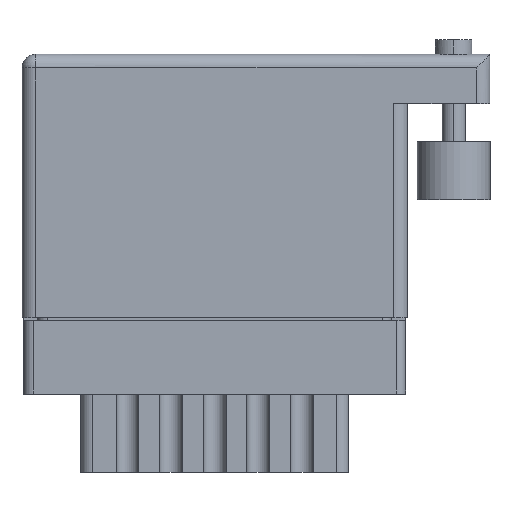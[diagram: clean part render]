
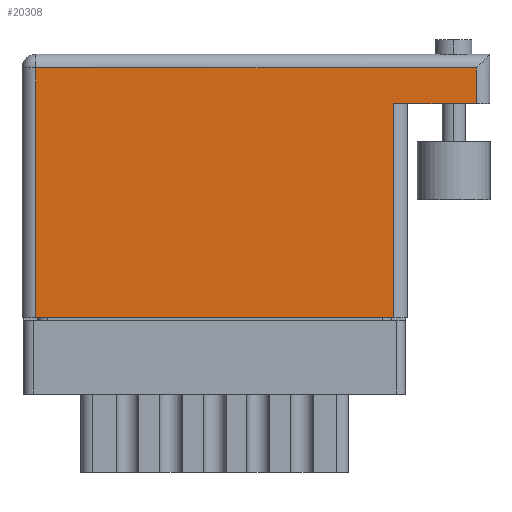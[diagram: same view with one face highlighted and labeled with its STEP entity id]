
A CAD part, front view. The second image highlights one B-rep face of the part: STEP entity #20308.
In plain terms, the highlighted face is planar.
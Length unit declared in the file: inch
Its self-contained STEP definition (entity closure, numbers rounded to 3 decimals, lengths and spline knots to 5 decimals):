
#1577 = VERTEX_POINT ( 'NONE', #13644 ) ;
#1664 = VECTOR ( 'NONE', #15111, 39.37008 ) ;
#1730 = EDGE_LOOP ( 'NONE', ( #14144, #26298, #18417, #25014, #15754, #8436 ) ) ;
#2524 = CARTESIAN_POINT ( 'NONE',  ( 1.562, 0.736, 0. ) ) ;
#3836 = VECTOR ( 'NONE', #26808, 39.37008 ) ;
#5490 = VERTEX_POINT ( 'NONE', #27435 ) ;
#5868 = EDGE_CURVE ( 'NONE', #21148, #5490, #8645, .T. ) ;
#6173 = VECTOR ( 'NONE', #8626, 39.37008 ) ;
#6643 = LINE ( 'NONE', #27378, #6173 ) ;
#7223 = DIRECTION ( 'NONE',  ( 1., 0., 0. ) ) ;
#8043 = CARTESIAN_POINT ( 'NONE',  ( 1.278, 0., 0. ) ) ;
#8205 = AXIS2_PLACEMENT_3D ( 'NONE', #13558, #23068, #22617 ) ;
#8436 = ORIENTED_EDGE ( 'NONE', *, *, #21082, .T. ) ;
#8458 = VERTEX_POINT ( 'NONE', #23476 ) ;
#8626 = DIRECTION ( 'NONE',  ( -1., 0., 0. ) ) ;
#8645 = LINE ( 'NONE', #11102, #1664 ) ;
#10105 = EDGE_CURVE ( 'NONE', #20045, #5490, #15119, .T. ) ;
#11102 = CARTESIAN_POINT ( 'NONE',  ( 1.278, 0.736, 0. ) ) ;
#12464 = EDGE_CURVE ( 'NONE', #20045, #15445, #19656, .T. ) ;
#13429 = CARTESIAN_POINT ( 'NONE',  ( 1.609, 0.736, 0. ) ) ;
#13558 = CARTESIAN_POINT ( 'NONE',  ( 0., 0.906, 0. ) ) ;
#13644 = CARTESIAN_POINT ( 'NONE',  ( 0.047, 0.859, 0. ) ) ;
#14144 = ORIENTED_EDGE ( 'NONE', *, *, #15978, .T. ) ;
#14521 = LINE ( 'NONE', #19103, #16553 ) ;
#15111 = DIRECTION ( 'NONE',  ( 0., 1., 0. ) ) ;
#15119 = LINE ( 'NONE', #13429, #3836 ) ;
#15199 = DIRECTION ( 'NONE',  ( 0., 1., 0. ) ) ;
#15445 = VERTEX_POINT ( 'NONE', #27748 ) ;
#15754 = ORIENTED_EDGE ( 'NONE', *, *, #19003, .T. ) ;
#15978 = EDGE_CURVE ( 'NONE', #8458, #21148, #18893, .T. ) ;
#16553 = VECTOR ( 'NONE', #23875, 39.37008 ) ;
#18417 = ORIENTED_EDGE ( 'NONE', *, *, #10105, .F. ) ;
#18893 = LINE ( 'NONE', #21350, #26365 ) ;
#19003 = EDGE_CURVE ( 'NONE', #15445, #1577, #6643, .T. ) ;
#19103 = CARTESIAN_POINT ( 'NONE',  ( 0.047, 0., 0. ) ) ;
#19656 = LINE ( 'NONE', #26889, #20714 ) ;
#20045 = VERTEX_POINT ( 'NONE', #2524 ) ;
#20308 = ADVANCED_FACE ( 'NONE', ( #20456 ), #29979, .F. ) ;
#20456 = FACE_OUTER_BOUND ( 'NONE', #1730, .T. ) ;
#20714 = VECTOR ( 'NONE', #15199, 39.37008 ) ;
#21082 = EDGE_CURVE ( 'NONE', #1577, #8458, #14521, .T. ) ;
#21148 = VERTEX_POINT ( 'NONE', #8043 ) ;
#21350 = CARTESIAN_POINT ( 'NONE',  ( 0., 0., 0. ) ) ;
#22617 = DIRECTION ( 'NONE',  ( -1., 0., 0. ) ) ;
#23068 = DIRECTION ( 'NONE',  ( 0., 0., -1. ) ) ;
#23476 = CARTESIAN_POINT ( 'NONE',  ( 0.047, 0., 0. ) ) ;
#23875 = DIRECTION ( 'NONE',  ( 0., -1., 0. ) ) ;
#25014 = ORIENTED_EDGE ( 'NONE', *, *, #12464, .T. ) ;
#26298 = ORIENTED_EDGE ( 'NONE', *, *, #5868, .T. ) ;
#26365 = VECTOR ( 'NONE', #7223, 39.37008 ) ;
#26808 = DIRECTION ( 'NONE',  ( -1., 0., 0. ) ) ;
#26889 = CARTESIAN_POINT ( 'NONE',  ( 1.562, 0.906, 0. ) ) ;
#27378 = CARTESIAN_POINT ( 'NONE',  ( 0., 0.859, 0. ) ) ;
#27435 = CARTESIAN_POINT ( 'NONE',  ( 1.278, 0.736, 0. ) ) ;
#27748 = CARTESIAN_POINT ( 'NONE',  ( 1.562, 0.859, 0. ) ) ;
#29979 = PLANE ( 'NONE',  #8205 ) ;
